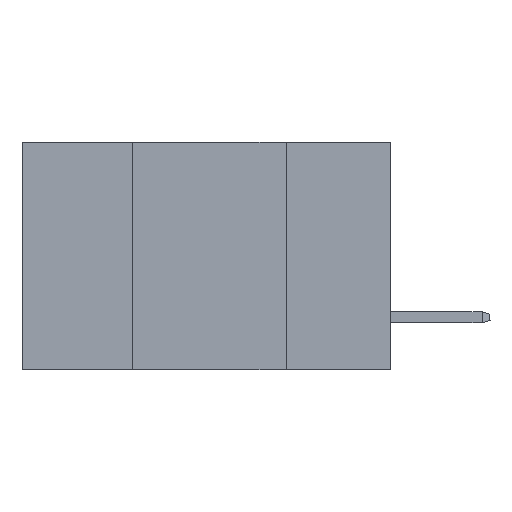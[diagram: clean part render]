
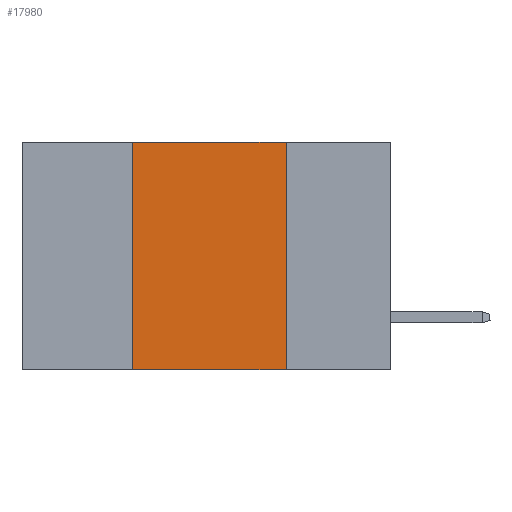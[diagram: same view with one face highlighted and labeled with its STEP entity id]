
A CAD part, left-side view. The second image highlights one B-rep face of the part: STEP entity #17980.
In plain terms, the highlighted planar face has unit normal (-1, 0, 0).
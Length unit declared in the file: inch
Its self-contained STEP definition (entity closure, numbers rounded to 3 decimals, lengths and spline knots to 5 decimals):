
#660 = ORIENTED_EDGE ( 'NONE', *, *, #19783, .F. ) ;
#800 = DIRECTION ( 'NONE',  ( 0., 0., -1. ) ) ;
#1248 = VECTOR ( 'NONE', #800, 39.37008 ) ;
#1290 = DIRECTION ( 'NONE',  ( 0., -1., 0. ) ) ;
#2644 = VECTOR ( 'NONE', #1290, 39.37008 ) ;
#3956 = CARTESIAN_POINT ( 'NONE',  ( 0., 0.42, -0.37 ) ) ;
#5639 = CARTESIAN_POINT ( 'NONE',  ( 0., 0.6, -0.37 ) ) ;
#5780 = VERTEX_POINT ( 'NONE', #3956 ) ;
#7427 = LINE ( 'NONE', #7806, #11400 ) ;
#7806 = CARTESIAN_POINT ( 'NONE',  ( 0., 0.6, 0. ) ) ;
#7840 = ORIENTED_EDGE ( 'NONE', *, *, #24773, .T. ) ;
#8112 = VECTOR ( 'NONE', #17201, 39.37008 ) ;
#9034 = CARTESIAN_POINT ( 'NONE',  ( 0., 0.42, 0. ) ) ;
#9040 = VERTEX_POINT ( 'NONE', #10941 ) ;
#9616 = VERTEX_POINT ( 'NONE', #25527 ) ;
#9665 = DIRECTION ( 'NONE',  ( 0., -1., 0. ) ) ;
#9808 = DIRECTION ( 'NONE',  ( 0., 0., -1. ) ) ;
#10286 = AXIS2_PLACEMENT_3D ( 'NONE', #15751, #15489, #9808 ) ;
#10941 = CARTESIAN_POINT ( 'NONE',  ( 0., 0.17, -0.37 ) ) ;
#11400 = VECTOR ( 'NONE', #9665, 39.37008 ) ;
#11412 = FACE_OUTER_BOUND ( 'NONE', #12790, .T. ) ;
#12733 = LINE ( 'NONE', #9034, #8112 ) ;
#12790 = EDGE_LOOP ( 'NONE', ( #660, #15247, #22254, #7840 ) ) ;
#15247 = ORIENTED_EDGE ( 'NONE', *, *, #22555, .F. ) ;
#15489 = DIRECTION ( 'NONE',  ( 1., 0., 0. ) ) ;
#15751 = CARTESIAN_POINT ( 'NONE',  ( 0., 0.6, 0. ) ) ;
#16682 = EDGE_CURVE ( 'NONE', #5780, #9616, #12733, .T. ) ;
#16952 = CARTESIAN_POINT ( 'NONE',  ( 0., 0.17, 0. ) ) ;
#17201 = DIRECTION ( 'NONE',  ( 0., 0., 1. ) ) ;
#17980 = ADVANCED_FACE ( 'NONE', ( #11412 ), #19471, .F. ) ;
#18892 = LINE ( 'NONE', #22834, #1248 ) ;
#19471 = PLANE ( 'NONE',  #10286 ) ;
#19783 = EDGE_CURVE ( 'NONE', #25048, #9040, #18892, .T. ) ;
#22254 = ORIENTED_EDGE ( 'NONE', *, *, #16682, .F. ) ;
#22555 = EDGE_CURVE ( 'NONE', #9616, #25048, #7427, .T. ) ;
#22834 = CARTESIAN_POINT ( 'NONE',  ( 0., 0.17, 0. ) ) ;
#23693 = LINE ( 'NONE', #5639, #2644 ) ;
#24773 = EDGE_CURVE ( 'NONE', #5780, #9040, #23693, .T. ) ;
#25048 = VERTEX_POINT ( 'NONE', #16952 ) ;
#25527 = CARTESIAN_POINT ( 'NONE',  ( 0., 0.42, 0. ) ) ;
